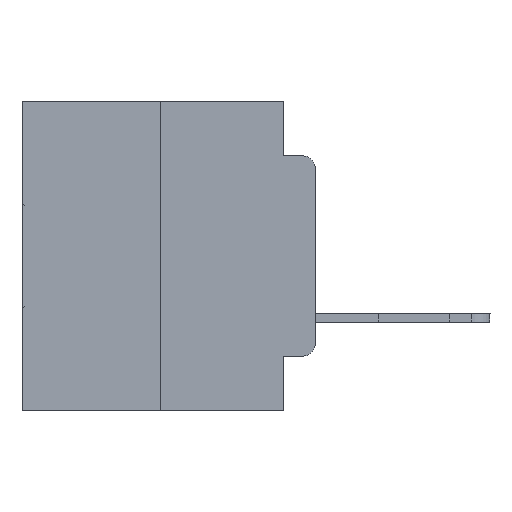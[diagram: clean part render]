
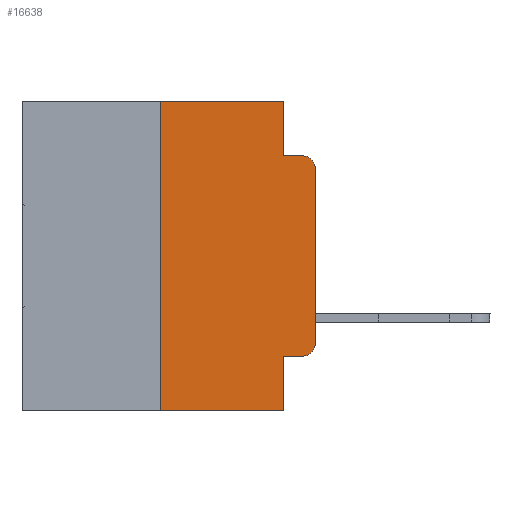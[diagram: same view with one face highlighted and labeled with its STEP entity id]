
A CAD part, left-side view. The second image highlights one B-rep face of the part: STEP entity #16638.
In plain terms, the highlighted planar face has unit normal (-1, 0, 0).
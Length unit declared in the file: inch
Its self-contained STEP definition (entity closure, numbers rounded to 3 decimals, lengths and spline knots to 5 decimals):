
#610 = DIRECTION ( 'NONE',  ( 0., 0., -1. ) ) ;
#677 = LINE ( 'NONE', #8610, #30332 ) ;
#952 = CARTESIAN_POINT ( 'NONE',  ( 0., 0.02, -0.4115 ) ) ;
#1147 = CARTESIAN_POINT ( 'NONE',  ( 0., 0.473, 0. ) ) ;
#1841 = DIRECTION ( 'NONE',  ( 0., 0., -1. ) ) ;
#1894 = EDGE_CURVE ( 'NONE', #14822, #9611, #22115, .T. ) ;
#2001 = LINE ( 'NONE', #13717, #14422 ) ;
#2059 = EDGE_CURVE ( 'NONE', #6190, #24856, #27892, .T. ) ;
#2077 = LINE ( 'NONE', #7023, #6382 ) ;
#2888 = EDGE_CURVE ( 'NONE', #23855, #6190, #18845, .T. ) ;
#3159 = AXIS2_PLACEMENT_3D ( 'NONE', #6774, #11350, #6294 ) ;
#3696 = FACE_OUTER_BOUND ( 'NONE', #30630, .T. ) ;
#4377 = ORIENTED_EDGE ( 'NONE', *, *, #18637, .F. ) ;
#5059 = VECTOR ( 'NONE', #7475, 39.37008 ) ;
#5261 = CARTESIAN_POINT ( 'NONE',  ( 0., 0., -0.1085 ) ) ;
#5620 = EDGE_CURVE ( 'NONE', #9611, #20748, #677, .T. ) ;
#6190 = VERTEX_POINT ( 'NONE', #952 ) ;
#6294 = DIRECTION ( 'NONE',  ( 0., 0., -1. ) ) ;
#6382 = VECTOR ( 'NONE', #9093, 39.37008 ) ;
#6607 = EDGE_CURVE ( 'NONE', #20748, #14045, #2001, .T. ) ;
#6774 = CARTESIAN_POINT ( 'NONE',  ( 0., 0.02, -0.3915 ) ) ;
#6778 = LINE ( 'NONE', #28266, #28930 ) ;
#7023 = CARTESIAN_POINT ( 'NONE',  ( 0., 0.473, -0.5 ) ) ;
#7475 = DIRECTION ( 'NONE',  ( 0., 0., -1. ) ) ;
#8610 = CARTESIAN_POINT ( 'NONE',  ( 0., 0.473, 0. ) ) ;
#8791 = AXIS2_PLACEMENT_3D ( 'NONE', #1147, #29226, #22252 ) ;
#9093 = DIRECTION ( 'NONE',  ( 0., -1., 0. ) ) ;
#9611 = VERTEX_POINT ( 'NONE', #12257 ) ;
#10134 = CARTESIAN_POINT ( 'NONE',  ( 0., 0.25, 0. ) ) ;
#10259 = PLANE ( 'NONE',  #8791 ) ;
#10678 = ORIENTED_EDGE ( 'NONE', *, *, #5620, .F. ) ;
#11205 = DIRECTION ( 'NONE',  ( 0., 0., 1. ) ) ;
#11345 = ORIENTED_EDGE ( 'NONE', *, *, #2888, .T. ) ;
#11350 = DIRECTION ( 'NONE',  ( -1., 0., 0. ) ) ;
#11613 = CARTESIAN_POINT ( 'NONE',  ( 0., 0.051, 0. ) ) ;
#12231 = ORIENTED_EDGE ( 'NONE', *, *, #16036, .T. ) ;
#12257 = CARTESIAN_POINT ( 'NONE',  ( 0., 0.25, 0. ) ) ;
#12933 = ORIENTED_EDGE ( 'NONE', *, *, #6607, .F. ) ;
#13717 = CARTESIAN_POINT ( 'NONE',  ( 0., 0.051, 0. ) ) ;
#14045 = VERTEX_POINT ( 'NONE', #21684 ) ;
#14323 = VERTEX_POINT ( 'NONE', #28296 ) ;
#14422 = VECTOR ( 'NONE', #1841, 39.37008 ) ;
#14499 = CIRCLE ( 'NONE', #21073, 0.02 ) ;
#14525 = ORIENTED_EDGE ( 'NONE', *, *, #1894, .F. ) ;
#14822 = VERTEX_POINT ( 'NONE', #28719 ) ;
#16036 = EDGE_CURVE ( 'NONE', #24856, #26595, #6778, .T. ) ;
#16184 = LINE ( 'NONE', #11613, #5059 ) ;
#16463 = CARTESIAN_POINT ( 'NONE',  ( 0., 0.051, -0.0885 ) ) ;
#16638 = ADVANCED_FACE ( 'NONE', ( #3696 ), #10259, .F. ) ;
#17457 = CARTESIAN_POINT ( 'NONE',  ( 0., 0., -0.3915 ) ) ;
#17951 = ORIENTED_EDGE ( 'NONE', *, *, #28331, .T. ) ;
#18637 = EDGE_CURVE ( 'NONE', #23855, #25922, #16184, .T. ) ;
#18845 = LINE ( 'NONE', #26577, #26752 ) ;
#20603 = DIRECTION ( 'NONE',  ( 0., -1., 0. ) ) ;
#20748 = VERTEX_POINT ( 'NONE', #27761 ) ;
#20800 = CARTESIAN_POINT ( 'NONE',  ( 0., 0.051, -0.5 ) ) ;
#21073 = AXIS2_PLACEMENT_3D ( 'NONE', #24654, #22288, #610 ) ;
#21428 = VECTOR ( 'NONE', #23576, 39.37008 ) ;
#21684 = CARTESIAN_POINT ( 'NONE',  ( 0., 0.051, -0.0885 ) ) ;
#22115 = LINE ( 'NONE', #10134, #28152 ) ;
#22252 = DIRECTION ( 'NONE',  ( 0., 0., -1. ) ) ;
#22288 = DIRECTION ( 'NONE',  ( -1., 0., 0. ) ) ;
#23486 = ORIENTED_EDGE ( 'NONE', *, *, #24318, .F. ) ;
#23576 = DIRECTION ( 'NONE',  ( 0., -1., 0. ) ) ;
#23745 = DIRECTION ( 'NONE',  ( 0., -1., 0. ) ) ;
#23855 = VERTEX_POINT ( 'NONE', #28832 ) ;
#24318 = EDGE_CURVE ( 'NONE', #14045, #14323, #25932, .T. ) ;
#24654 = CARTESIAN_POINT ( 'NONE',  ( 0., 0.02, -0.1085 ) ) ;
#24856 = VERTEX_POINT ( 'NONE', #17457 ) ;
#25922 = VERTEX_POINT ( 'NONE', #20800 ) ;
#25932 = LINE ( 'NONE', #16463, #21428 ) ;
#26163 = ORIENTED_EDGE ( 'NONE', *, *, #26492, .T. ) ;
#26492 = EDGE_CURVE ( 'NONE', #14822, #25922, #2077, .T. ) ;
#26577 = CARTESIAN_POINT ( 'NONE',  ( 0., 0.051, -0.4115 ) ) ;
#26595 = VERTEX_POINT ( 'NONE', #5261 ) ;
#26752 = VECTOR ( 'NONE', #23745, 39.37008 ) ;
#27761 = CARTESIAN_POINT ( 'NONE',  ( 0., 0.051, 0. ) ) ;
#27892 = CIRCLE ( 'NONE', #3159, 0.02 ) ;
#28152 = VECTOR ( 'NONE', #29395, 39.37008 ) ;
#28266 = CARTESIAN_POINT ( 'NONE',  ( 0., 0., 0. ) ) ;
#28296 = CARTESIAN_POINT ( 'NONE',  ( 0., 0.02, -0.0885 ) ) ;
#28331 = EDGE_CURVE ( 'NONE', #26595, #14323, #14499, .T. ) ;
#28719 = CARTESIAN_POINT ( 'NONE',  ( 0., 0.25, -0.5 ) ) ;
#28832 = CARTESIAN_POINT ( 'NONE',  ( 0., 0.051, -0.4115 ) ) ;
#28930 = VECTOR ( 'NONE', #11205, 39.37008 ) ;
#29226 = DIRECTION ( 'NONE',  ( 1., 0., 0. ) ) ;
#29395 = DIRECTION ( 'NONE',  ( 0., 0., 1. ) ) ;
#30332 = VECTOR ( 'NONE', #20603, 39.37008 ) ;
#30577 = ORIENTED_EDGE ( 'NONE', *, *, #2059, .T. ) ;
#30630 = EDGE_LOOP ( 'NONE', ( #12231, #17951, #23486, #12933, #10678, #14525, #26163, #4377, #11345, #30577 ) ) ;
